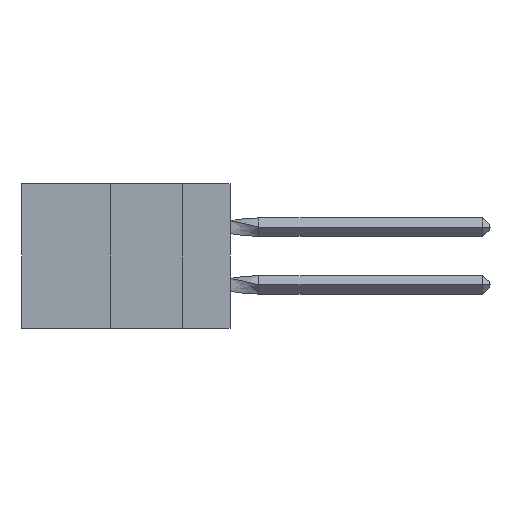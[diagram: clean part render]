
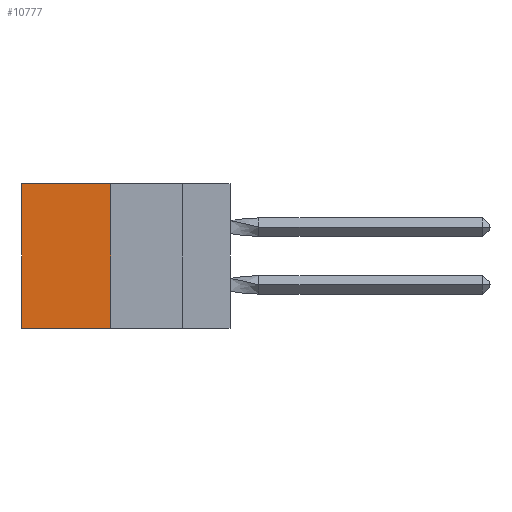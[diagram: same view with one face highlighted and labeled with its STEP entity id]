
A CAD part, left-side view. The second image highlights one B-rep face of the part: STEP entity #10777.
In plain terms, the highlighted planar face has unit normal (-1, 0, 0).
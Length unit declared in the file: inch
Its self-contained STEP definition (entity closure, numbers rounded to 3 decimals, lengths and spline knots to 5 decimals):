
#2112 = ORIENTED_EDGE ( 'NONE', *, *, #4875, .T. ) ;
#3376 = CARTESIAN_POINT ( 'NONE',  ( 0.305, 0.413, -0.5 ) ) ;
#3766 = DIRECTION ( 'NONE',  ( 1., 0., 0. ) ) ;
#3867 = LINE ( 'NONE', #34976, #36410 ) ;
#4151 = CARTESIAN_POINT ( 'NONE',  ( 0.305, 0.72, -0.5 ) ) ;
#4875 = EDGE_CURVE ( 'NONE', #24528, #13166, #6948, .T. ) ;
#5828 = CARTESIAN_POINT ( 'NONE',  ( 0.305, 0.72, 0. ) ) ;
#6948 = LINE ( 'NONE', #4151, #15016 ) ;
#7259 = DIRECTION ( 'NONE',  ( 0., 0., -1. ) ) ;
#10076 = ORIENTED_EDGE ( 'NONE', *, *, #24976, .T. ) ;
#10282 = DIRECTION ( 'NONE',  ( 0., 0., -1. ) ) ;
#10777 = ADVANCED_FACE ( 'NONE', ( #17270 ), #22055, .F. ) ;
#11543 = EDGE_CURVE ( 'NONE', #38477, #20656, #3867, .T. ) ;
#12316 = LINE ( 'NONE', #3376, #35810 ) ;
#13166 = VERTEX_POINT ( 'NONE', #37173 ) ;
#13253 = CARTESIAN_POINT ( 'NONE',  ( 0.305, 0.413, 0. ) ) ;
#13941 = EDGE_LOOP ( 'NONE', ( #2112, #29912, #23040, #10076 ) ) ;
#15016 = VECTOR ( 'NONE', #10282, 39.37008 ) ;
#17270 = FACE_OUTER_BOUND ( 'NONE', #13941, .T. ) ;
#20041 = VECTOR ( 'NONE', #25682, 39.37008 ) ;
#20656 = VERTEX_POINT ( 'NONE', #31123 ) ;
#21935 = CARTESIAN_POINT ( 'NONE',  ( 0.305, 0.413, -0.5 ) ) ;
#22055 = PLANE ( 'NONE',  #35335 ) ;
#23040 = ORIENTED_EDGE ( 'NONE', *, *, #11543, .F. ) ;
#24528 = VERTEX_POINT ( 'NONE', #5828 ) ;
#24976 = EDGE_CURVE ( 'NONE', #38477, #24528, #32478, .T. ) ;
#25682 = DIRECTION ( 'NONE',  ( 0., 1., 0. ) ) ;
#25745 = EDGE_CURVE ( 'NONE', #20656, #13166, #12316, .T. ) ;
#27547 = DIRECTION ( 'NONE',  ( 0., 1., 0. ) ) ;
#29912 = ORIENTED_EDGE ( 'NONE', *, *, #25745, .F. ) ;
#31123 = CARTESIAN_POINT ( 'NONE',  ( 0.305, 0.413, -0.5 ) ) ;
#32334 = CARTESIAN_POINT ( 'NONE',  ( 0.305, 0.413, 0. ) ) ;
#32478 = LINE ( 'NONE', #13253, #20041 ) ;
#33858 = DIRECTION ( 'NONE',  ( 0., 0., -1. ) ) ;
#34976 = CARTESIAN_POINT ( 'NONE',  ( 0.305, 0.413, -0.5 ) ) ;
#35335 = AXIS2_PLACEMENT_3D ( 'NONE', #21935, #3766, #33858 ) ;
#35810 = VECTOR ( 'NONE', #27547, 39.37008 ) ;
#36410 = VECTOR ( 'NONE', #7259, 39.37008 ) ;
#37173 = CARTESIAN_POINT ( 'NONE',  ( 0.305, 0.72, -0.5 ) ) ;
#38477 = VERTEX_POINT ( 'NONE', #32334 ) ;
